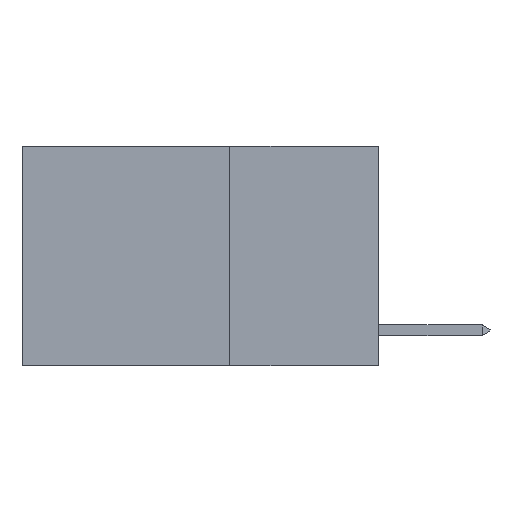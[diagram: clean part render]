
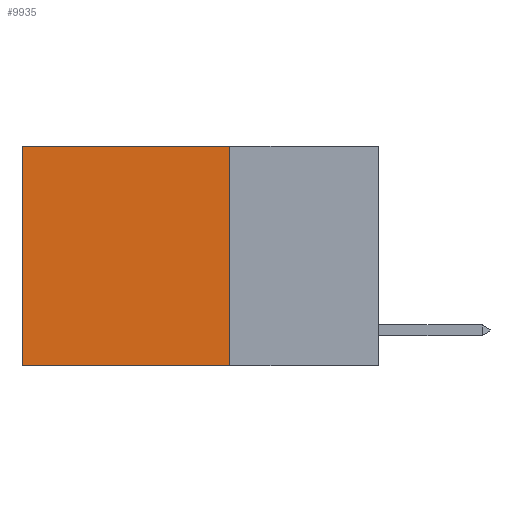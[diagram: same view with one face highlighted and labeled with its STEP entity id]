
A CAD part, left-side view. The second image highlights one B-rep face of the part: STEP entity #9935.
In plain terms, the highlighted planar face has unit normal (-1, 0, 0).
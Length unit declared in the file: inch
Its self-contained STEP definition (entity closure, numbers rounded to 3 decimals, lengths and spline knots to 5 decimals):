
#272 = EDGE_CURVE ( 'NONE', #14454, #1204, #16555, .T. ) ;
#1107 = DIRECTION ( 'NONE',  ( 0., 0., -1. ) ) ;
#1204 = VERTEX_POINT ( 'NONE', #11728 ) ;
#2078 = LINE ( 'NONE', #3747, #10427 ) ;
#3080 = CARTESIAN_POINT ( 'NONE',  ( 0.2625, 0.6, 0. ) ) ;
#3105 = EDGE_CURVE ( 'NONE', #4680, #14454, #2078, .T. ) ;
#3620 = ORIENTED_EDGE ( 'NONE', *, *, #11647, .T. ) ;
#3724 = DIRECTION ( 'NONE',  ( 0., 1., 0. ) ) ;
#3747 = CARTESIAN_POINT ( 'NONE',  ( 0.2625, 0.25, 0. ) ) ;
#4680 = VERTEX_POINT ( 'NONE', #10158 ) ;
#5016 = FACE_OUTER_BOUND ( 'NONE', #10078, .T. ) ;
#7116 = VECTOR ( 'NONE', #3724, 39.37008 ) ;
#7154 = LINE ( 'NONE', #17556, #9903 ) ;
#7227 = ORIENTED_EDGE ( 'NONE', *, *, #15024, .T. ) ;
#9062 = ORIENTED_EDGE ( 'NONE', *, *, #3105, .F. ) ;
#9903 = VECTOR ( 'NONE', #13015, 39.37008 ) ;
#9935 = ADVANCED_FACE ( 'NONE', ( #5016 ), #16071, .F. ) ;
#10078 = EDGE_LOOP ( 'NONE', ( #3620, #16657, #9062, #7227 ) ) ;
#10148 = DIRECTION ( 'NONE',  ( 1., 0., 0. ) ) ;
#10158 = CARTESIAN_POINT ( 'NONE',  ( 0.2625, 0.25, 0. ) ) ;
#10427 = VECTOR ( 'NONE', #17225, 39.37008 ) ;
#10464 = CARTESIAN_POINT ( 'NONE',  ( 0.2625, 0.6, 0. ) ) ;
#11647 = EDGE_CURVE ( 'NONE', #13564, #1204, #13525, .T. ) ;
#11728 = CARTESIAN_POINT ( 'NONE',  ( 0.2625, 0.6, -0.37 ) ) ;
#11750 = CARTESIAN_POINT ( 'NONE',  ( 0.2625, 0.25, 0. ) ) ;
#11855 = DIRECTION ( 'NONE',  ( 0., 0., -1. ) ) ;
#13015 = DIRECTION ( 'NONE',  ( 0., 1., 0. ) ) ;
#13525 = LINE ( 'NONE', #10464, #17696 ) ;
#13564 = VERTEX_POINT ( 'NONE', #3080 ) ;
#14454 = VERTEX_POINT ( 'NONE', #19399 ) ;
#15024 = EDGE_CURVE ( 'NONE', #4680, #13564, #7154, .T. ) ;
#16071 = PLANE ( 'NONE',  #16544 ) ;
#16544 = AXIS2_PLACEMENT_3D ( 'NONE', #11750, #10148, #1107 ) ;
#16555 = LINE ( 'NONE', #17735, #7116 ) ;
#16657 = ORIENTED_EDGE ( 'NONE', *, *, #272, .F. ) ;
#17225 = DIRECTION ( 'NONE',  ( 0., 0., -1. ) ) ;
#17556 = CARTESIAN_POINT ( 'NONE',  ( 0.2625, 0.25, 0. ) ) ;
#17696 = VECTOR ( 'NONE', #11855, 39.37008 ) ;
#17735 = CARTESIAN_POINT ( 'NONE',  ( 0.2625, 0.25, -0.37 ) ) ;
#19399 = CARTESIAN_POINT ( 'NONE',  ( 0.2625, 0.25, -0.37 ) ) ;
